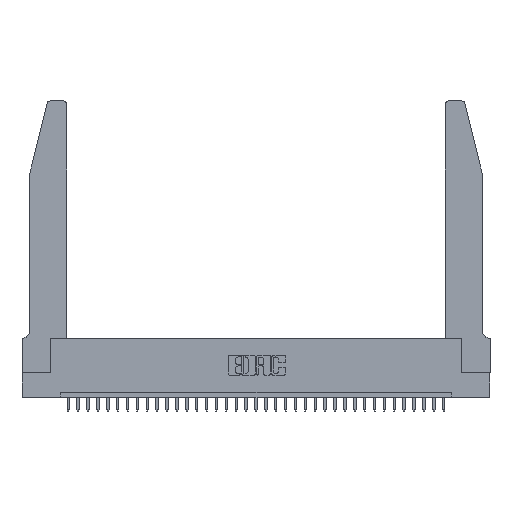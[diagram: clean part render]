
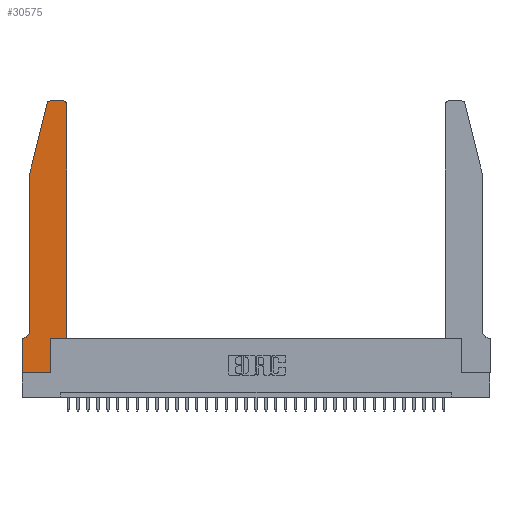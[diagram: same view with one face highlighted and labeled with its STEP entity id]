
A CAD part, top view. The second image highlights one B-rep face of the part: STEP entity #30575.
In plain terms, the highlighted planar face has unit normal (0, 0, 1).
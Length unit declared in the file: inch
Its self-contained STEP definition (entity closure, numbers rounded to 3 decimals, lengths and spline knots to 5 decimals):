
#346 = CARTESIAN_POINT ( 'NONE',  ( 0.25487, 2.72718, 0.37 ) ) ;
#851 = ORIENTED_EDGE ( 'NONE', *, *, #12596, .T. ) ;
#880 = AXIS2_PLACEMENT_3D ( 'NONE', #33718, #17524, #14756 ) ;
#963 = CARTESIAN_POINT ( 'NONE',  ( 0.0755, 0.35, 0.37 ) ) ;
#1060 = CARTESIAN_POINT ( 'NONE',  ( 0.2865, 0.35, 0.37 ) ) ;
#1146 = LINE ( 'NONE', #22321, #4936 ) ;
#1464 = EDGE_CURVE ( 'NONE', #32041, #25585, #5504, .T. ) ;
#1509 = DIRECTION ( 'NONE',  ( 0., 1., 0. ) ) ;
#1536 = ORIENTED_EDGE ( 'NONE', *, *, #2091, .T. ) ;
#1900 = VERTEX_POINT ( 'NONE', #28956 ) ;
#2091 = EDGE_CURVE ( 'NONE', #9739, #1900, #24604, .T. ) ;
#2160 = VECTOR ( 'NONE', #28376, 39.37008 ) ;
#2217 = LINE ( 'NONE', #25208, #8918 ) ;
#2309 = AXIS2_PLACEMENT_3D ( 'NONE', #32783, #19641, #8683 ) ;
#2708 = CARTESIAN_POINT ( 'NONE',  ( 0.2605, 2.75, 0.37 ) ) ;
#3035 = VERTEX_POINT ( 'NONE', #3963 ) ;
#3072 = EDGE_CURVE ( 'NONE', #7046, #3035, #33727, .T. ) ;
#3295 = VECTOR ( 'NONE', #3643, 39.37008 ) ;
#3643 = DIRECTION ( 'NONE',  ( -1., 0., 0. ) ) ;
#3963 = CARTESIAN_POINT ( 'NONE',  ( 0.284, 2.75, 0.37 ) ) ;
#4397 = CARTESIAN_POINT ( 'NONE',  ( 0.2865, 0.35, 0.37 ) ) ;
#4463 = ORIENTED_EDGE ( 'NONE', *, *, #29295, .T. ) ;
#4936 = VECTOR ( 'NONE', #20576, 39.37008 ) ;
#5504 = LINE ( 'NONE', #27989, #22583 ) ;
#6091 = VECTOR ( 'NONE', #10586, 39.37008 ) ;
#6159 = DIRECTION ( 'NONE',  ( 0., 0., 1. ) ) ;
#6182 = CARTESIAN_POINT ( 'NONE',  ( 0.284, 2.72, 0.37 ) ) ;
#7046 = VERTEX_POINT ( 'NONE', #11508 ) ;
#7459 = DIRECTION ( 'NONE',  ( 1., 0., 0. ) ) ;
#8123 = LINE ( 'NONE', #25612, #32686 ) ;
#8683 = DIRECTION ( 'NONE',  ( -1., 0., 0. ) ) ;
#8859 = DIRECTION ( 'NONE',  ( 0., 0., 1. ) ) ;
#8918 = VECTOR ( 'NONE', #22877, 39.37008 ) ;
#8997 = EDGE_CURVE ( 'NONE', #32874, #32391, #17669, .T. ) ;
#9475 = CARTESIAN_POINT ( 'NONE',  ( 0.0755, 2., 0.37 ) ) ;
#9739 = VERTEX_POINT ( 'NONE', #32359 ) ;
#10207 = EDGE_LOOP ( 'NONE', ( #31224, #851, #20636, #33271, #31057, #1536, #14604, #19061, #31941, #16478, #14922, #4463 ) ) ;
#10341 = LINE ( 'NONE', #21267, #6091 ) ;
#10586 = DIRECTION ( 'NONE',  ( 0., -1., 0. ) ) ;
#11508 = CARTESIAN_POINT ( 'NONE',  ( 0.4205, 2.75, 0.37 ) ) ;
#11555 = DIRECTION ( 'NONE',  ( 1., 0., 0. ) ) ;
#11589 = FACE_OUTER_BOUND ( 'NONE', #10207, .T. ) ;
#12596 = EDGE_CURVE ( 'NONE', #3035, #23635, #28564, .T. ) ;
#12652 = LINE ( 'NONE', #4397, #2160 ) ;
#13507 = CIRCLE ( 'NONE', #880, 0.03 ) ;
#14333 = CARTESIAN_POINT ( 'NONE',  ( 0.0755, 0.42, 0.37 ) ) ;
#14446 = VERTEX_POINT ( 'NONE', #27170 ) ;
#14604 = ORIENTED_EDGE ( 'NONE', *, *, #27598, .T. ) ;
#14756 = DIRECTION ( 'NONE',  ( 1., 0., 0. ) ) ;
#14922 = ORIENTED_EDGE ( 'NONE', *, *, #1464, .T. ) ;
#15533 = CARTESIAN_POINT ( 'NONE',  ( 0.4505, 0.35, 0.37 ) ) ;
#15773 = CARTESIAN_POINT ( 'NONE',  ( 0.4505, 2.72, 0.37 ) ) ;
#16478 = ORIENTED_EDGE ( 'NONE', *, *, #28703, .T. ) ;
#17524 = DIRECTION ( 'NONE',  ( 0., 0., 1. ) ) ;
#17669 = LINE ( 'NONE', #9475, #33512 ) ;
#18720 = CARTESIAN_POINT ( 'NONE',  ( 0.0755, 2., 0.37 ) ) ;
#19061 = ORIENTED_EDGE ( 'NONE', *, *, #25993, .T. ) ;
#19081 = AXIS2_PLACEMENT_3D ( 'NONE', #6182, #8859, #11555 ) ;
#19641 = DIRECTION ( 'NONE',  ( 0., 0., -1. ) ) ;
#20210 = AXIS2_PLACEMENT_3D ( 'NONE', #30124, #6159, #21979 ) ;
#20576 = DIRECTION ( 'NONE',  ( 1., 0., 0. ) ) ;
#20636 = ORIENTED_EDGE ( 'NONE', *, *, #21050, .T. ) ;
#20744 = VERTEX_POINT ( 'NONE', #22869 ) ;
#21050 = EDGE_CURVE ( 'NONE', #23635, #32874, #2217, .T. ) ;
#21267 = CARTESIAN_POINT ( 'NONE',  ( 0., 0., 0.37 ) ) ;
#21979 = DIRECTION ( 'NONE',  ( 1., 0., 0. ) ) ;
#22321 = CARTESIAN_POINT ( 'NONE',  ( 0., 0., 0.37 ) ) ;
#22583 = VECTOR ( 'NONE', #1509, 39.37008 ) ;
#22810 = CIRCLE ( 'NONE', #2309, 0.07 ) ;
#22844 = VERTEX_POINT ( 'NONE', #1060 ) ;
#22869 = CARTESIAN_POINT ( 'NONE',  ( 0.2865, 0., 0.37 ) ) ;
#22877 = DIRECTION ( 'NONE',  ( -0.239, -0.971, 0. ) ) ;
#23635 = VERTEX_POINT ( 'NONE', #346 ) ;
#23735 = VECTOR ( 'NONE', #27058, 39.37008 ) ;
#24604 = LINE ( 'NONE', #963, #3295 ) ;
#25208 = CARTESIAN_POINT ( 'NONE',  ( 0.0755, 2., 0.37 ) ) ;
#25585 = VERTEX_POINT ( 'NONE', #15773 ) ;
#25612 = CARTESIAN_POINT ( 'NONE',  ( 0.4505, 0.35, 0.37 ) ) ;
#25993 = EDGE_CURVE ( 'NONE', #14446, #20744, #1146, .T. ) ;
#27058 = DIRECTION ( 'NONE',  ( -1., 0., 0. ) ) ;
#27170 = CARTESIAN_POINT ( 'NONE',  ( 0., 0., 0.37 ) ) ;
#27598 = EDGE_CURVE ( 'NONE', #1900, #14446, #10341, .T. ) ;
#27723 = DIRECTION ( 'NONE',  ( 0., -1., 0. ) ) ;
#27989 = CARTESIAN_POINT ( 'NONE',  ( 0.4505, 0.35, 0.37 ) ) ;
#28376 = DIRECTION ( 'NONE',  ( 0., 1., 0. ) ) ;
#28564 = CIRCLE ( 'NONE', #19081, 0.03 ) ;
#28703 = EDGE_CURVE ( 'NONE', #22844, #32041, #8123, .T. ) ;
#28956 = CARTESIAN_POINT ( 'NONE',  ( 0., 0.35, 0.37 ) ) ;
#29295 = EDGE_CURVE ( 'NONE', #25585, #7046, #13507, .T. ) ;
#30004 = PLANE ( 'NONE',  #20210 ) ;
#30124 = CARTESIAN_POINT ( 'NONE',  ( 0., 0.35, 0.37 ) ) ;
#30575 = ADVANCED_FACE ( 'NONE', ( #11589 ), #30004, .T. ) ;
#31057 = ORIENTED_EDGE ( 'NONE', *, *, #31140, .T. ) ;
#31140 = EDGE_CURVE ( 'NONE', #32391, #9739, #22810, .T. ) ;
#31224 = ORIENTED_EDGE ( 'NONE', *, *, #3072, .T. ) ;
#31941 = ORIENTED_EDGE ( 'NONE', *, *, #33915, .T. ) ;
#32041 = VERTEX_POINT ( 'NONE', #15533 ) ;
#32359 = CARTESIAN_POINT ( 'NONE',  ( 0.0055, 0.35, 0.37 ) ) ;
#32391 = VERTEX_POINT ( 'NONE', #14333 ) ;
#32686 = VECTOR ( 'NONE', #7459, 39.37008 ) ;
#32783 = CARTESIAN_POINT ( 'NONE',  ( 0.0055, 0.42, 0.37 ) ) ;
#32874 = VERTEX_POINT ( 'NONE', #18720 ) ;
#33271 = ORIENTED_EDGE ( 'NONE', *, *, #8997, .T. ) ;
#33512 = VECTOR ( 'NONE', #27723, 39.37008 ) ;
#33718 = CARTESIAN_POINT ( 'NONE',  ( 0.4205, 2.72, 0.37 ) ) ;
#33727 = LINE ( 'NONE', #2708, #23735 ) ;
#33915 = EDGE_CURVE ( 'NONE', #20744, #22844, #12652, .T. ) ;
